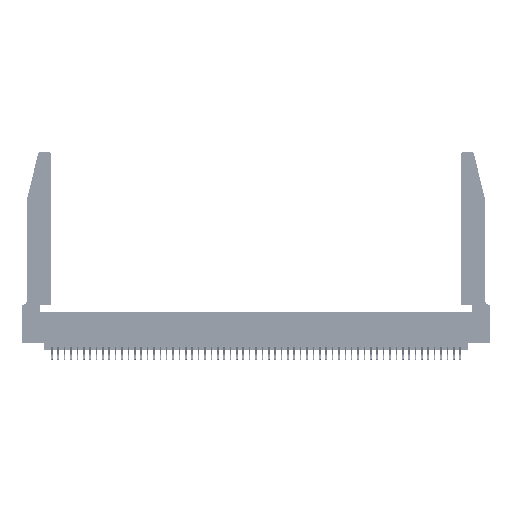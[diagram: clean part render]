
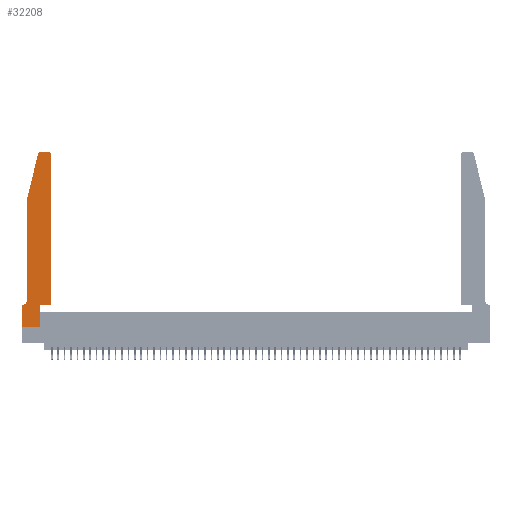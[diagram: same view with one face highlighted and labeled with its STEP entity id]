
A CAD part, top view. The second image highlights one B-rep face of the part: STEP entity #32208.
In plain terms, the highlighted planar face has unit normal (0, 0, 1).
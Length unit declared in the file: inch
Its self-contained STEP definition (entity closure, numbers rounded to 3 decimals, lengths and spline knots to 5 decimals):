
#444 = VERTEX_POINT ( 'NONE', #50747 ) ;
#1132 = ORIENTED_EDGE ( 'NONE', *, *, #15004, .T. ) ;
#1556 = ORIENTED_EDGE ( 'NONE', *, *, #44970, .T. ) ;
#2383 = DIRECTION ( 'NONE',  ( 0., 0., -1. ) ) ;
#2633 = CARTESIAN_POINT ( 'NONE',  ( 0., 0.35, 0.37 ) ) ;
#2760 = VERTEX_POINT ( 'NONE', #15413 ) ;
#2808 = DIRECTION ( 'NONE',  ( 1., 0., 0. ) ) ;
#2976 = ORIENTED_EDGE ( 'NONE', *, *, #36546, .T. ) ;
#4055 = VERTEX_POINT ( 'NONE', #4119 ) ;
#4119 = CARTESIAN_POINT ( 'NONE',  ( 0.0755, 2., 0.37 ) ) ;
#4167 = AXIS2_PLACEMENT_3D ( 'NONE', #2633, #31261, #2808 ) ;
#4815 = CARTESIAN_POINT ( 'NONE',  ( 0.2865, 0., 0.37 ) ) ;
#4859 = CARTESIAN_POINT ( 'NONE',  ( 0.0755, 0.35, 0.37 ) ) ;
#6812 = LINE ( 'NONE', #27977, #34359 ) ;
#7011 = DIRECTION ( 'NONE',  ( 0., 0., 1. ) ) ;
#7743 = CARTESIAN_POINT ( 'NONE',  ( 0., 0.35, 0.37 ) ) ;
#8506 = VECTOR ( 'NONE', #23883, 39.37008 ) ;
#8821 = EDGE_CURVE ( 'NONE', #27274, #34504, #43738, .T. ) ;
#8852 = EDGE_CURVE ( 'NONE', #4055, #43012, #41186, .T. ) ;
#9672 = ORIENTED_EDGE ( 'NONE', *, *, #12597, .T. ) ;
#12405 = CARTESIAN_POINT ( 'NONE',  ( 0.4205, 2.72, 0.37 ) ) ;
#12438 = FACE_OUTER_BOUND ( 'NONE', #49170, .T. ) ;
#12597 = EDGE_CURVE ( 'NONE', #42985, #46421, #46209, .T. ) ;
#13933 = CARTESIAN_POINT ( 'NONE',  ( 0.0755, 2., 0.37 ) ) ;
#14204 = DIRECTION ( 'NONE',  ( -1., 0., 0. ) ) ;
#15004 = EDGE_CURVE ( 'NONE', #2760, #27274, #38903, .T. ) ;
#15413 = CARTESIAN_POINT ( 'NONE',  ( 0.0055, 0.35, 0.37 ) ) ;
#15471 = CARTESIAN_POINT ( 'NONE',  ( 0., 0., 0.37 ) ) ;
#16164 = EDGE_CURVE ( 'NONE', #444, #42985, #29159, .T. ) ;
#17234 = EDGE_CURVE ( 'NONE', #45700, #48615, #33529, .T. ) ;
#18307 = VECTOR ( 'NONE', #38957, 39.37008 ) ;
#18803 = VECTOR ( 'NONE', #51022, 39.37008 ) ;
#19067 = AXIS2_PLACEMENT_3D ( 'NONE', #46955, #2383, #14204 ) ;
#19383 = VECTOR ( 'NONE', #36028, 39.37008 ) ;
#20372 = VECTOR ( 'NONE', #45027, 39.37008 ) ;
#20561 = ORIENTED_EDGE ( 'NONE', *, *, #8852, .T. ) ;
#22115 = CARTESIAN_POINT ( 'NONE',  ( 0.284, 2.75, 0.37 ) ) ;
#23347 = DIRECTION ( 'NONE',  ( 0., 1., 0. ) ) ;
#23435 = VERTEX_POINT ( 'NONE', #45160 ) ;
#23883 = DIRECTION ( 'NONE',  ( 0., -1., 0. ) ) ;
#24372 = EDGE_CURVE ( 'NONE', #46421, #4055, #45787, .T. ) ;
#26757 = EDGE_CURVE ( 'NONE', #48615, #23435, #36994, .T. ) ;
#26770 = CIRCLE ( 'NONE', #19067, 0.07 ) ;
#27233 = DIRECTION ( 'NONE',  ( 1., 0., 0. ) ) ;
#27274 = VERTEX_POINT ( 'NONE', #7743 ) ;
#27327 = CARTESIAN_POINT ( 'NONE',  ( 0.2865, 0.35, 0.37 ) ) ;
#27977 = CARTESIAN_POINT ( 'NONE',  ( 0.4505, 0.35, 0.37 ) ) ;
#29156 = VECTOR ( 'NONE', #42936, 39.37008 ) ;
#29159 = LINE ( 'NONE', #30510, #18307 ) ;
#29260 = EDGE_CURVE ( 'NONE', #50841, #444, #32903, .T. ) ;
#29355 = DIRECTION ( 'NONE',  ( -1., 0., 0. ) ) ;
#29840 = ORIENTED_EDGE ( 'NONE', *, *, #24372, .T. ) ;
#30510 = CARTESIAN_POINT ( 'NONE',  ( 0.2605, 2.75, 0.37 ) ) ;
#31184 = CARTESIAN_POINT ( 'NONE',  ( 0.4505, 2.72, 0.37 ) ) ;
#31261 = DIRECTION ( 'NONE',  ( 0., 0., 1. ) ) ;
#31330 = ORIENTED_EDGE ( 'NONE', *, *, #26757, .T. ) ;
#32208 = ADVANCED_FACE ( 'NONE', ( #12438 ), #43805, .T. ) ;
#32802 = DIRECTION ( 'NONE',  ( 1., 0., 0. ) ) ;
#32852 = AXIS2_PLACEMENT_3D ( 'NONE', #12405, #49465, #48310 ) ;
#32903 = CIRCLE ( 'NONE', #32852, 0.03 ) ;
#33387 = CARTESIAN_POINT ( 'NONE',  ( 0., 0., 0.37 ) ) ;
#33529 = LINE ( 'NONE', #38678, #18803 ) ;
#34359 = VECTOR ( 'NONE', #23347, 39.37008 ) ;
#34504 = VERTEX_POINT ( 'NONE', #33387 ) ;
#34583 = ORIENTED_EDGE ( 'NONE', *, *, #16164, .T. ) ;
#35153 = CARTESIAN_POINT ( 'NONE',  ( 0.0755, 0.42, 0.37 ) ) ;
#35676 = CARTESIAN_POINT ( 'NONE',  ( 0.0755, 2., 0.37 ) ) ;
#36028 = DIRECTION ( 'NONE',  ( 0., -1., 0. ) ) ;
#36546 = EDGE_CURVE ( 'NONE', #43012, #2760, #26770, .T. ) ;
#36994 = LINE ( 'NONE', #49162, #20372 ) ;
#38678 = CARTESIAN_POINT ( 'NONE',  ( 0.2865, 0.35, 0.37 ) ) ;
#38903 = LINE ( 'NONE', #4859, #51070 ) ;
#38957 = DIRECTION ( 'NONE',  ( -1., 0., 0. ) ) ;
#40158 = ORIENTED_EDGE ( 'NONE', *, *, #8821, .T. ) ;
#41084 = AXIS2_PLACEMENT_3D ( 'NONE', #51793, #7011, #27233 ) ;
#41186 = LINE ( 'NONE', #35676, #19383 ) ;
#41372 = EDGE_CURVE ( 'NONE', #23435, #50841, #6812, .T. ) ;
#42855 = ORIENTED_EDGE ( 'NONE', *, *, #29260, .T. ) ;
#42936 = DIRECTION ( 'NONE',  ( -0.239, -0.971, 0. ) ) ;
#42985 = VERTEX_POINT ( 'NONE', #22115 ) ;
#43012 = VERTEX_POINT ( 'NONE', #35153 ) ;
#43397 = LINE ( 'NONE', #52866, #49831 ) ;
#43738 = LINE ( 'NONE', #15471, #8506 ) ;
#43805 = PLANE ( 'NONE',  #4167 ) ;
#44555 = ORIENTED_EDGE ( 'NONE', *, *, #17234, .T. ) ;
#44970 = EDGE_CURVE ( 'NONE', #34504, #45700, #43397, .T. ) ;
#45027 = DIRECTION ( 'NONE',  ( 1., 0., 0. ) ) ;
#45160 = CARTESIAN_POINT ( 'NONE',  ( 0.4505, 0.35, 0.37 ) ) ;
#45700 = VERTEX_POINT ( 'NONE', #4815 ) ;
#45787 = LINE ( 'NONE', #13933, #29156 ) ;
#46209 = CIRCLE ( 'NONE', #41084, 0.03 ) ;
#46421 = VERTEX_POINT ( 'NONE', #49511 ) ;
#46955 = CARTESIAN_POINT ( 'NONE',  ( 0.0055, 0.42, 0.37 ) ) ;
#48310 = DIRECTION ( 'NONE',  ( 1., 0., 0. ) ) ;
#48615 = VERTEX_POINT ( 'NONE', #27327 ) ;
#49162 = CARTESIAN_POINT ( 'NONE',  ( 0.4505, 0.35, 0.37 ) ) ;
#49170 = EDGE_LOOP ( 'NONE', ( #34583, #9672, #29840, #20561, #2976, #1132, #40158, #1556, #44555, #31330, #49488, #42855 ) ) ;
#49465 = DIRECTION ( 'NONE',  ( 0., 0., 1. ) ) ;
#49488 = ORIENTED_EDGE ( 'NONE', *, *, #41372, .T. ) ;
#49511 = CARTESIAN_POINT ( 'NONE',  ( 0.25487, 2.72718, 0.37 ) ) ;
#49831 = VECTOR ( 'NONE', #32802, 39.37008 ) ;
#50747 = CARTESIAN_POINT ( 'NONE',  ( 0.4205, 2.75, 0.37 ) ) ;
#50841 = VERTEX_POINT ( 'NONE', #31184 ) ;
#51022 = DIRECTION ( 'NONE',  ( 0., 1., 0. ) ) ;
#51070 = VECTOR ( 'NONE', #29355, 39.37008 ) ;
#51793 = CARTESIAN_POINT ( 'NONE',  ( 0.284, 2.72, 0.37 ) ) ;
#52866 = CARTESIAN_POINT ( 'NONE',  ( 0., 0., 0.37 ) ) ;
